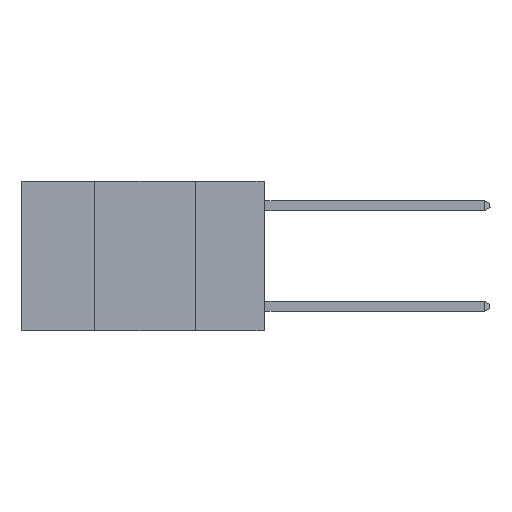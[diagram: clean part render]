
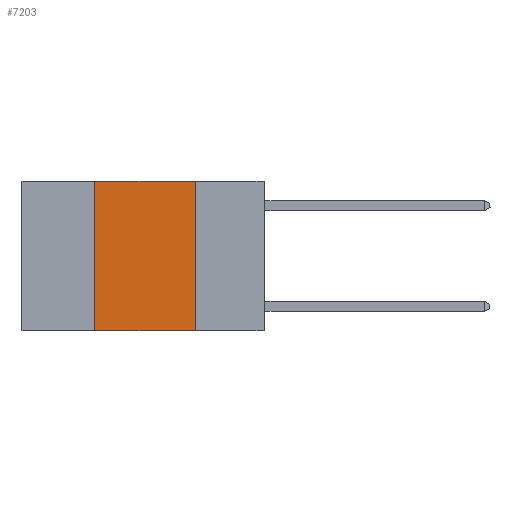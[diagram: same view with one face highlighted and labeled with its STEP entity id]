
A CAD part, left-side view. The second image highlights one B-rep face of the part: STEP entity #7203.
In plain terms, the highlighted planar face has unit normal (-1, 0, 0).
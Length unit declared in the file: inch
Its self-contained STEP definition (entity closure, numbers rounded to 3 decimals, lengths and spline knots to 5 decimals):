
#131 = ORIENTED_EDGE ( 'NONE', *, *, #3602, .F. ) ;
#250 = PLANE ( 'NONE',  #10980 ) ;
#440 = CARTESIAN_POINT ( 'NONE',  ( 0., 0.6, 0. ) ) ;
#1131 = ORIENTED_EDGE ( 'NONE', *, *, #7689, .T. ) ;
#1333 = EDGE_CURVE ( 'NONE', #12577, #14994, #6397, .T. ) ;
#2453 = VECTOR ( 'NONE', #5430, 39.37008 ) ;
#2753 = DIRECTION ( 'NONE',  ( 0., 0., -1. ) ) ;
#3223 = CARTESIAN_POINT ( 'NONE',  ( 0., 0.6, -0.37 ) ) ;
#3361 = DIRECTION ( 'NONE',  ( 0., 0., 1. ) ) ;
#3602 = EDGE_CURVE ( 'NONE', #3705, #4435, #9179, .T. ) ;
#3705 = VERTEX_POINT ( 'NONE', #10285 ) ;
#4081 = VECTOR ( 'NONE', #4519, 39.37008 ) ;
#4435 = VERTEX_POINT ( 'NONE', #5426 ) ;
#4474 = LINE ( 'NONE', #3223, #4081 ) ;
#4519 = DIRECTION ( 'NONE',  ( 0., -1., 0. ) ) ;
#5426 = CARTESIAN_POINT ( 'NONE',  ( 0., 0.42, 0. ) ) ;
#5430 = DIRECTION ( 'NONE',  ( 0., -1., 0. ) ) ;
#5623 = EDGE_LOOP ( 'NONE', ( #6772, #15012, #131, #1131 ) ) ;
#5716 = LINE ( 'NONE', #440, #2453 ) ;
#6397 = LINE ( 'NONE', #15208, #12441 ) ;
#6772 = ORIENTED_EDGE ( 'NONE', *, *, #1333, .F. ) ;
#7203 = ADVANCED_FACE ( 'NONE', ( #10817 ), #250, .F. ) ;
#7689 = EDGE_CURVE ( 'NONE', #3705, #14994, #4474, .T. ) ;
#8215 = EDGE_CURVE ( 'NONE', #4435, #12577, #5716, .T. ) ;
#8720 = DIRECTION ( 'NONE',  ( 0., 0., -1. ) ) ;
#8759 = CARTESIAN_POINT ( 'NONE',  ( 0., 0.6, 0. ) ) ;
#8807 = VECTOR ( 'NONE', #3361, 39.37008 ) ;
#9179 = LINE ( 'NONE', #14324, #8807 ) ;
#9980 = DIRECTION ( 'NONE',  ( 1., 0., 0. ) ) ;
#10285 = CARTESIAN_POINT ( 'NONE',  ( 0., 0.42, -0.37 ) ) ;
#10817 = FACE_OUTER_BOUND ( 'NONE', #5623, .T. ) ;
#10980 = AXIS2_PLACEMENT_3D ( 'NONE', #8759, #9980, #2753 ) ;
#12024 = CARTESIAN_POINT ( 'NONE',  ( 0., 0.17, -0.37 ) ) ;
#12441 = VECTOR ( 'NONE', #8720, 39.37008 ) ;
#12577 = VERTEX_POINT ( 'NONE', #15313 ) ;
#14324 = CARTESIAN_POINT ( 'NONE',  ( 0., 0.42, 0. ) ) ;
#14994 = VERTEX_POINT ( 'NONE', #12024 ) ;
#15012 = ORIENTED_EDGE ( 'NONE', *, *, #8215, .F. ) ;
#15208 = CARTESIAN_POINT ( 'NONE',  ( 0., 0.17, 0. ) ) ;
#15313 = CARTESIAN_POINT ( 'NONE',  ( 0., 0.17, 0. ) ) ;
